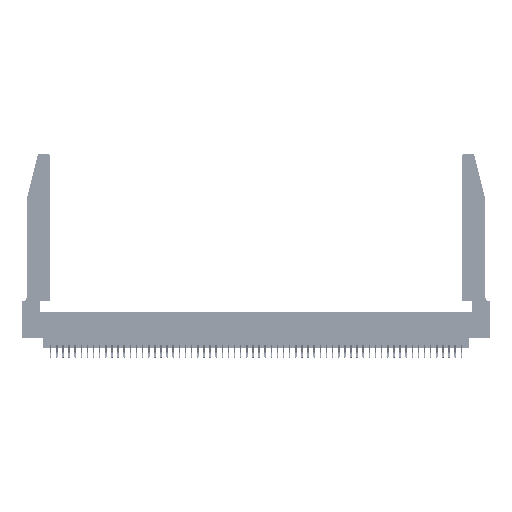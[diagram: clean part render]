
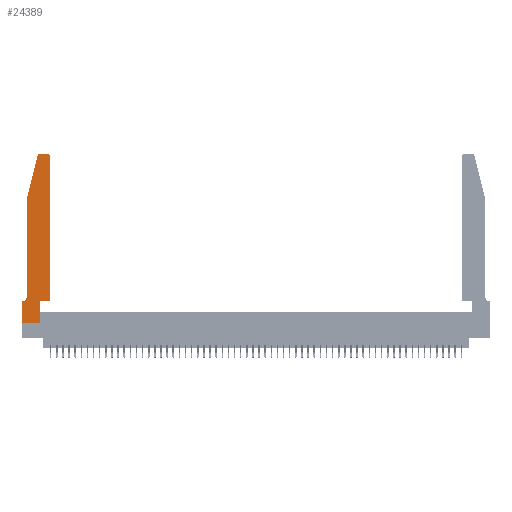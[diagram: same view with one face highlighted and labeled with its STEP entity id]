
A CAD part, top view. The second image highlights one B-rep face of the part: STEP entity #24389.
In plain terms, the highlighted planar face has unit normal (0, 0, 1).
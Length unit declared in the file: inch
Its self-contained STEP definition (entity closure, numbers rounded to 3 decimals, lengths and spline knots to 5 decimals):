
#302 = CARTESIAN_POINT ( 'NONE',  ( 0.0755, 0.42, 0.37 ) ) ;
#1258 = VERTEX_POINT ( 'NONE', #24499 ) ;
#1265 = CARTESIAN_POINT ( 'NONE',  ( 0.0755, 2., 0.37 ) ) ;
#1350 = CIRCLE ( 'NONE', #23221, 0.03 ) ;
#1548 = EDGE_CURVE ( 'NONE', #3409, #5199, #7865, .T. ) ;
#1783 = ORIENTED_EDGE ( 'NONE', *, *, #45970, .T. ) ;
#2216 = CARTESIAN_POINT ( 'NONE',  ( 0., 0., 0.37 ) ) ;
#2413 = LINE ( 'NONE', #26702, #34058 ) ;
#3409 = VERTEX_POINT ( 'NONE', #48770 ) ;
#4153 = LINE ( 'NONE', #2216, #16925 ) ;
#5199 = VERTEX_POINT ( 'NONE', #30520 ) ;
#6582 = VECTOR ( 'NONE', #47440, 39.37008 ) ;
#6792 = ORIENTED_EDGE ( 'NONE', *, *, #32251, .T. ) ;
#7201 = CIRCLE ( 'NONE', #20369, 0.07 ) ;
#7637 = AXIS2_PLACEMENT_3D ( 'NONE', #16124, #45746, #20414 ) ;
#7761 = LINE ( 'NONE', #39766, #50176 ) ;
#7865 = LINE ( 'NONE', #22629, #40400 ) ;
#8313 = CIRCLE ( 'NONE', #7637, 0.03 ) ;
#8803 = CARTESIAN_POINT ( 'NONE',  ( 0.284, 2.75, 0.37 ) ) ;
#9209 = ORIENTED_EDGE ( 'NONE', *, *, #21998, .T. ) ;
#9720 = ORIENTED_EDGE ( 'NONE', *, *, #11988, .T. ) ;
#10271 = DIRECTION ( 'NONE',  ( -0.239, -0.971, 0. ) ) ;
#10401 = VECTOR ( 'NONE', #25029, 39.37008 ) ;
#11988 = EDGE_CURVE ( 'NONE', #24899, #24318, #8313, .T. ) ;
#13025 = VECTOR ( 'NONE', #24747, 39.37008 ) ;
#13159 = CARTESIAN_POINT ( 'NONE',  ( 0.25487, 2.72718, 0.37 ) ) ;
#13598 = CARTESIAN_POINT ( 'NONE',  ( 0.0055, 0.42, 0.37 ) ) ;
#13915 = PLANE ( 'NONE',  #46383 ) ;
#14291 = DIRECTION ( 'NONE',  ( -1., 0., 0. ) ) ;
#14368 = ORIENTED_EDGE ( 'NONE', *, *, #34863, .T. ) ;
#14492 = FACE_OUTER_BOUND ( 'NONE', #40807, .T. ) ;
#16124 = CARTESIAN_POINT ( 'NONE',  ( 0.284, 2.72, 0.37 ) ) ;
#16498 = CARTESIAN_POINT ( 'NONE',  ( 0.2865, 0.35, 0.37 ) ) ;
#16925 = VECTOR ( 'NONE', #32049, 39.37008 ) ;
#17881 = DIRECTION ( 'NONE',  ( -1., 0., 0. ) ) ;
#17969 = DIRECTION ( 'NONE',  ( 0., 0., 1. ) ) ;
#19717 = VERTEX_POINT ( 'NONE', #1265 ) ;
#19867 = DIRECTION ( 'NONE',  ( 0., -1., 0. ) ) ;
#20311 = EDGE_CURVE ( 'NONE', #52256, #3409, #7201, .T. ) ;
#20369 = AXIS2_PLACEMENT_3D ( 'NONE', #13598, #43215, #17881 ) ;
#20414 = DIRECTION ( 'NONE',  ( 1., 0., 0. ) ) ;
#21546 = CARTESIAN_POINT ( 'NONE',  ( 0., 0., 0.37 ) ) ;
#21998 = EDGE_CURVE ( 'NONE', #1258, #52915, #44238, .T. ) ;
#22629 = CARTESIAN_POINT ( 'NONE',  ( 0.0755, 0.35, 0.37 ) ) ;
#23221 = AXIS2_PLACEMENT_3D ( 'NONE', #43307, #17969, #47552 ) ;
#24158 = ORIENTED_EDGE ( 'NONE', *, *, #32188, .T. ) ;
#24285 = LINE ( 'NONE', #29048, #45471 ) ;
#24318 = VERTEX_POINT ( 'NONE', #13159 ) ;
#24389 = ADVANCED_FACE ( 'NONE', ( #14492 ), #13915, .T. ) ;
#24499 = CARTESIAN_POINT ( 'NONE',  ( 0.2865, 0., 0.37 ) ) ;
#24712 = ORIENTED_EDGE ( 'NONE', *, *, #31828, .T. ) ;
#24747 = DIRECTION ( 'NONE',  ( 1., 0., 0. ) ) ;
#24899 = VERTEX_POINT ( 'NONE', #8803 ) ;
#25029 = DIRECTION ( 'NONE',  ( 0., 1., 0. ) ) ;
#25326 = EDGE_CURVE ( 'NONE', #52915, #31902, #46835, .T. ) ;
#26702 = CARTESIAN_POINT ( 'NONE',  ( 0.4505, 0.35, 0.37 ) ) ;
#26747 = DIRECTION ( 'NONE',  ( 1., 0., 0. ) ) ;
#28992 = ORIENTED_EDGE ( 'NONE', *, *, #33544, .T. ) ;
#29048 = CARTESIAN_POINT ( 'NONE',  ( 0., 0., 0.37 ) ) ;
#29233 = LINE ( 'NONE', #43189, #6582 ) ;
#30520 = CARTESIAN_POINT ( 'NONE',  ( 0., 0.35, 0.37 ) ) ;
#31234 = VERTEX_POINT ( 'NONE', #45070 ) ;
#31828 = EDGE_CURVE ( 'NONE', #19717, #52256, #43977, .T. ) ;
#31902 = VERTEX_POINT ( 'NONE', #45757 ) ;
#32049 = DIRECTION ( 'NONE',  ( 0., -1., 0. ) ) ;
#32188 = EDGE_CURVE ( 'NONE', #40120, #31234, #1350, .T. ) ;
#32251 = EDGE_CURVE ( 'NONE', #31902, #40120, #2413, .T. ) ;
#33289 = DIRECTION ( 'NONE',  ( 1., 0., 0. ) ) ;
#33544 = EDGE_CURVE ( 'NONE', #31234, #24899, #29233, .T. ) ;
#34058 = VECTOR ( 'NONE', #43677, 39.37008 ) ;
#34162 = ORIENTED_EDGE ( 'NONE', *, *, #41922, .T. ) ;
#34863 = EDGE_CURVE ( 'NONE', #24318, #19717, #7761, .T. ) ;
#36760 = CARTESIAN_POINT ( 'NONE',  ( 0.0755, 2., 0.37 ) ) ;
#39766 = CARTESIAN_POINT ( 'NONE',  ( 0.0755, 2., 0.37 ) ) ;
#40120 = VERTEX_POINT ( 'NONE', #48386 ) ;
#40400 = VECTOR ( 'NONE', #14291, 39.37008 ) ;
#40807 = EDGE_LOOP ( 'NONE', ( #28992, #9720, #14368, #24712, #41988, #41396, #1783, #34162, #9209, #54562, #6792, #24158 ) ) ;
#41396 = ORIENTED_EDGE ( 'NONE', *, *, #1548, .T. ) ;
#41922 = EDGE_CURVE ( 'NONE', #44055, #1258, #24285, .T. ) ;
#41988 = ORIENTED_EDGE ( 'NONE', *, *, #20311, .T. ) ;
#43165 = CARTESIAN_POINT ( 'NONE',  ( 0., 0.35, 0.37 ) ) ;
#43189 = CARTESIAN_POINT ( 'NONE',  ( 0.2605, 2.75, 0.37 ) ) ;
#43215 = DIRECTION ( 'NONE',  ( 0., 0., -1. ) ) ;
#43307 = CARTESIAN_POINT ( 'NONE',  ( 0.4205, 2.72, 0.37 ) ) ;
#43677 = DIRECTION ( 'NONE',  ( 0., 1., 0. ) ) ;
#43977 = LINE ( 'NONE', #36760, #53878 ) ;
#44055 = VERTEX_POINT ( 'NONE', #21546 ) ;
#44238 = LINE ( 'NONE', #16498, #10401 ) ;
#45070 = CARTESIAN_POINT ( 'NONE',  ( 0.4205, 2.75, 0.37 ) ) ;
#45471 = VECTOR ( 'NONE', #33289, 39.37008 ) ;
#45746 = DIRECTION ( 'NONE',  ( 0., 0., 1. ) ) ;
#45757 = CARTESIAN_POINT ( 'NONE',  ( 0.4505, 0.35, 0.37 ) ) ;
#45854 = CARTESIAN_POINT ( 'NONE',  ( 0.4505, 0.35, 0.37 ) ) ;
#45970 = EDGE_CURVE ( 'NONE', #5199, #44055, #4153, .T. ) ;
#46383 = AXIS2_PLACEMENT_3D ( 'NONE', #43165, #52016, #26747 ) ;
#46835 = LINE ( 'NONE', #45854, #13025 ) ;
#46907 = CARTESIAN_POINT ( 'NONE',  ( 0.2865, 0.35, 0.37 ) ) ;
#47440 = DIRECTION ( 'NONE',  ( -1., 0., 0. ) ) ;
#47552 = DIRECTION ( 'NONE',  ( 1., 0., 0. ) ) ;
#48386 = CARTESIAN_POINT ( 'NONE',  ( 0.4505, 2.72, 0.37 ) ) ;
#48770 = CARTESIAN_POINT ( 'NONE',  ( 0.0055, 0.35, 0.37 ) ) ;
#50176 = VECTOR ( 'NONE', #10271, 39.37008 ) ;
#52016 = DIRECTION ( 'NONE',  ( 0., 0., 1. ) ) ;
#52256 = VERTEX_POINT ( 'NONE', #302 ) ;
#52915 = VERTEX_POINT ( 'NONE', #46907 ) ;
#53878 = VECTOR ( 'NONE', #19867, 39.37008 ) ;
#54562 = ORIENTED_EDGE ( 'NONE', *, *, #25326, .T. ) ;
